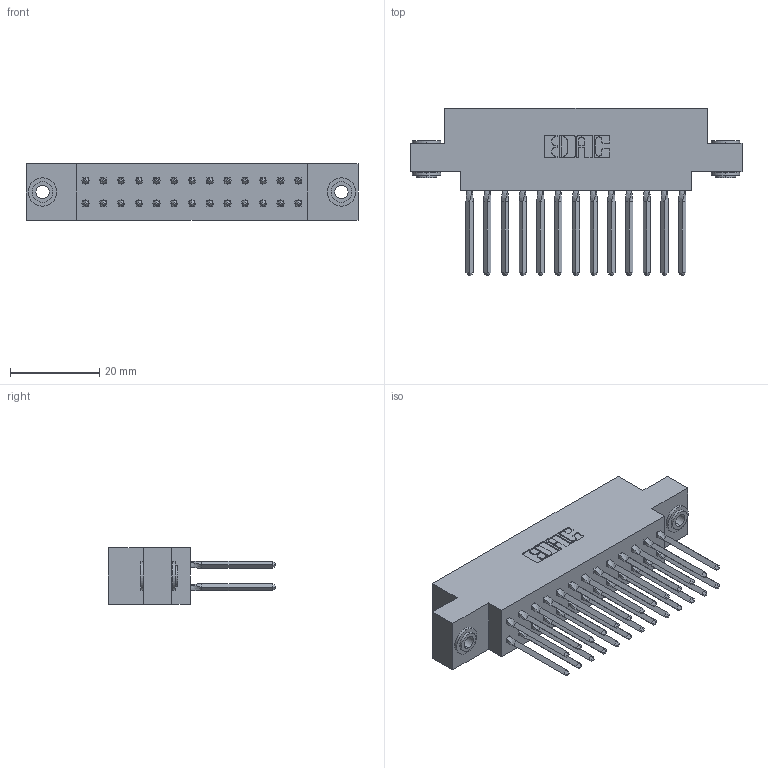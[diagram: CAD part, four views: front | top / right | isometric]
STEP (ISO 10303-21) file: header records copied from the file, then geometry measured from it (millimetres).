
FILE_DESCRIPTION (( 'STEP AP203' ), '1' );
FILE_NAME ('317-026-540-803.STEP', '2020-02-27T18:48:59', ( '' ), ( '' ), 'SwSTEP 2.0', 'SolidWorks 2016', '' );
FILE_SCHEMA (( 'CONFIG_CONTROL_DESIGN' ));
Length unit declared in the file: inch
Products named in the file (4): 317-290-001_540; 345-250-002_345-250-002-102; 317 Part_.156 Dia - TH; 317-026-540-803
Assembly tree (29 placements, depth 2):
  317-026-540-803
    317 Part_.156 Dia - TH
    317-290-001_540  x26
    345-250-002_345-250-002-102  x2
Bounding box: 74.22 x 37.34 x 12.7 mm (x, y, z)
Volume: 11495.1 mm3; surface area: 16256.1 mm2
Topology: 29 solids, 29 shells, 2454 faces, 6773 edges, 4364 vertices
Faces by surface type: plane 1966, cylinder 376, bspline 104, cone 8
Entity records: 23487 total; most frequent: CARTESIAN_POINT 4478, ORIENTED_EDGE 3970, DIRECTION 3357, EDGE_CURVE 1985, LINE 1705, VECTOR 1705, VERTEX_POINT 1315, AXIS2_PLACEMENT_3D 826
